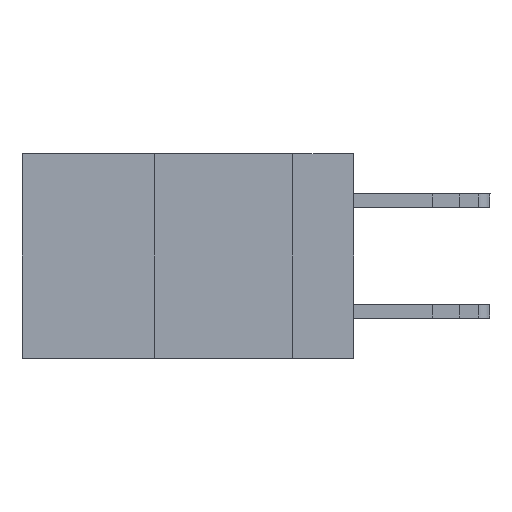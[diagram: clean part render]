
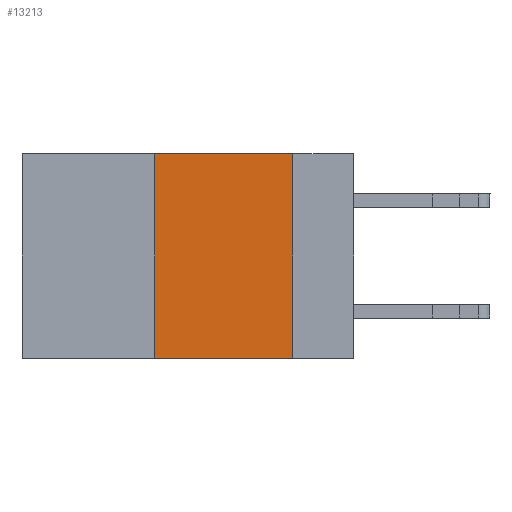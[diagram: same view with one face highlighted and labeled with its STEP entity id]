
A CAD part, left-side view. The second image highlights one B-rep face of the part: STEP entity #13213.
In plain terms, the highlighted planar face has unit normal (-1, 0, 0).
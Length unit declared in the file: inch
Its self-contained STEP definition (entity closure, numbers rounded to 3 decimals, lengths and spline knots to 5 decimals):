
#149 = CARTESIAN_POINT ( 'NONE',  ( 0., 0.11, 0. ) ) ;
#891 = ORIENTED_EDGE ( 'NONE', *, *, #15943, .F. ) ;
#1199 = VERTEX_POINT ( 'NONE', #18659 ) ;
#1313 = CARTESIAN_POINT ( 'NONE',  ( 0., 0.11, -0.37 ) ) ;
#1930 = ORIENTED_EDGE ( 'NONE', *, *, #13687, .F. ) ;
#2073 = DIRECTION ( 'NONE',  ( 1., 0., 0. ) ) ;
#2218 = EDGE_CURVE ( 'NONE', #13443, #18455, #18905, .T. ) ;
#2503 = ORIENTED_EDGE ( 'NONE', *, *, #2218, .F. ) ;
#3189 = CARTESIAN_POINT ( 'NONE',  ( 0., 0.36, 0. ) ) ;
#3483 = LINE ( 'NONE', #3189, #7410 ) ;
#3788 = CARTESIAN_POINT ( 'NONE',  ( 0., 0.6, 0. ) ) ;
#4046 = CARTESIAN_POINT ( 'NONE',  ( 0., 0.6, 0. ) ) ;
#7410 = VECTOR ( 'NONE', #14222, 39.37008 ) ;
#7990 = CARTESIAN_POINT ( 'NONE',  ( 0., 0.11, 0. ) ) ;
#8156 = FACE_OUTER_BOUND ( 'NONE', #9673, .T. ) ;
#8253 = DIRECTION ( 'NONE',  ( 0., 0., -1. ) ) ;
#8403 = DIRECTION ( 'NONE',  ( 0., -1., 0. ) ) ;
#8828 = EDGE_CURVE ( 'NONE', #1199, #18455, #11730, .T. ) ;
#9673 = EDGE_LOOP ( 'NONE', ( #2503, #1930, #891, #16040 ) ) ;
#10348 = PLANE ( 'NONE',  #19885 ) ;
#11173 = DIRECTION ( 'NONE',  ( 0., 0., -1. ) ) ;
#11730 = LINE ( 'NONE', #17937, #14182 ) ;
#12225 = CARTESIAN_POINT ( 'NONE',  ( 0., 0.36, 0. ) ) ;
#13213 = ADVANCED_FACE ( 'NONE', ( #8156 ), #10348, .F. ) ;
#13443 = VERTEX_POINT ( 'NONE', #7990 ) ;
#13504 = VECTOR ( 'NONE', #8403, 39.37008 ) ;
#13687 = EDGE_CURVE ( 'NONE', #19961, #13443, #16102, .T. ) ;
#14182 = VECTOR ( 'NONE', #16499, 39.37008 ) ;
#14222 = DIRECTION ( 'NONE',  ( 0., 0., 1. ) ) ;
#15509 = VECTOR ( 'NONE', #11173, 39.37008 ) ;
#15943 = EDGE_CURVE ( 'NONE', #1199, #19961, #3483, .T. ) ;
#16040 = ORIENTED_EDGE ( 'NONE', *, *, #8828, .T. ) ;
#16102 = LINE ( 'NONE', #4046, #13504 ) ;
#16499 = DIRECTION ( 'NONE',  ( 0., -1., 0. ) ) ;
#17937 = CARTESIAN_POINT ( 'NONE',  ( 0., 0.6, -0.37 ) ) ;
#18455 = VERTEX_POINT ( 'NONE', #1313 ) ;
#18659 = CARTESIAN_POINT ( 'NONE',  ( 0., 0.36, -0.37 ) ) ;
#18905 = LINE ( 'NONE', #149, #15509 ) ;
#19885 = AXIS2_PLACEMENT_3D ( 'NONE', #3788, #2073, #8253 ) ;
#19961 = VERTEX_POINT ( 'NONE', #12225 ) ;
